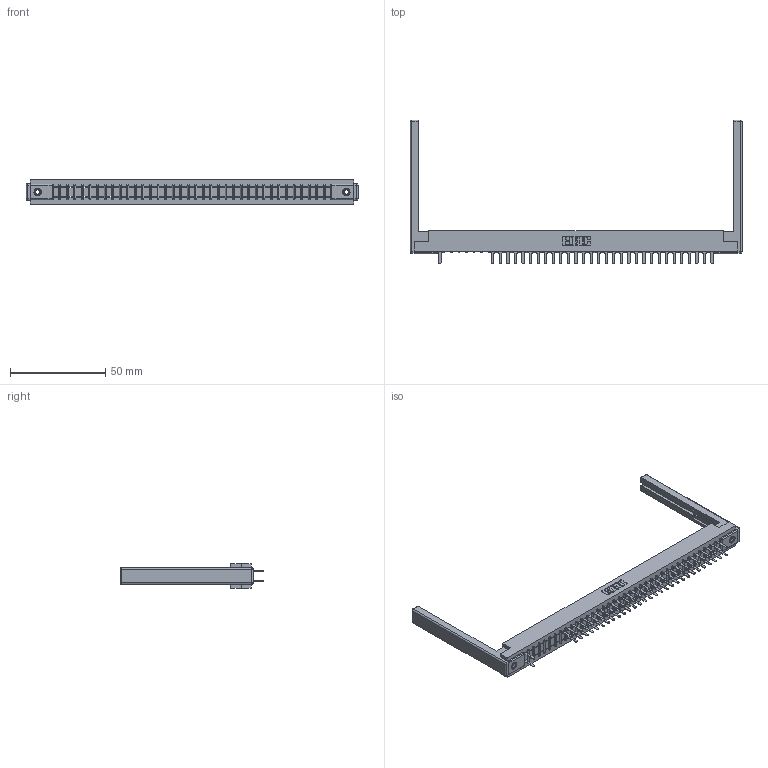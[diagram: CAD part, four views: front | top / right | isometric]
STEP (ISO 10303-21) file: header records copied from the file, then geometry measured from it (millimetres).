
FILE_DESCRIPTION (( 'STEP AP203' ), '1' );
FILE_NAME ('307-074-520-268.STEP', '2018-08-06T16:01:24', ( '' ), ( '' ), 'SwSTEP 2.0', 'SolidWorks 2016', '' );
FILE_SCHEMA (( 'CONFIG_CONTROL_DESIGN' ));
Length unit declared in the file: inch
Products named in the file (5): 307 Part_.156 Dia Mounting Holes; 307-290-001_520; 307-220-068; 345-250-001_345-250-001-102; 307-074-520-268
Assembly tree (66 placements, depth 2):
  307-074-520-268
    307 Part_.156 Dia Mounting Holes
    307-290-001_520  x61
    307-220-068  x2
    345-250-001_345-250-001-102  x2
Bounding box: 174.04 x 75.39 x 12.7 mm (x, y, z)
Volume: 22728.7 mm3; surface area: 25323.8 mm2
Topology: 66 solids, 66 shells, 3246 faces, 9059 edges, 5834 vertices
Faces by surface type: plane 2127, cylinder 1019, sphere 84, cone 12, torus 4
Entity records: 35831 total; most frequent: CARTESIAN_POINT 5893, ORIENTED_EDGE 5844, DIRECTION 5776, EDGE_CURVE 2922, VECTOR 2238, LINE 2238, VERTEX_POINT 1886, AXIS2_PLACEMENT_3D 1769
